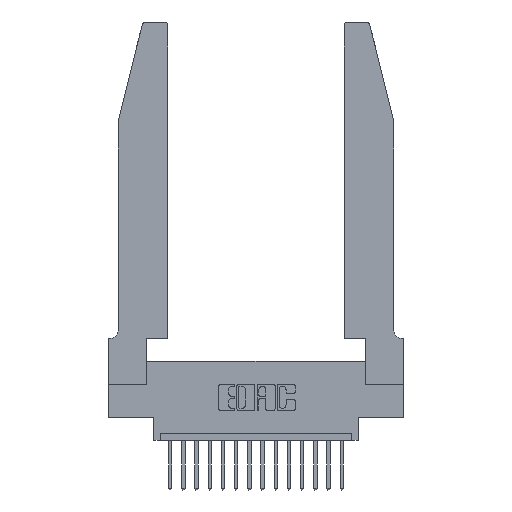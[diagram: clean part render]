
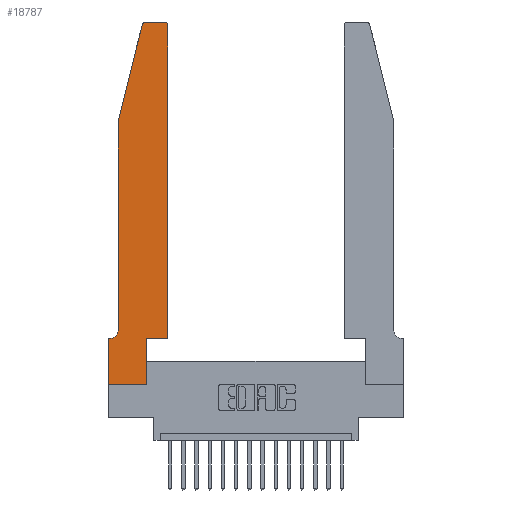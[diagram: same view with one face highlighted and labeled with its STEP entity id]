
A CAD part, top view. The second image highlights one B-rep face of the part: STEP entity #18787.
In plain terms, the highlighted planar face has unit normal (0, 0, 1).
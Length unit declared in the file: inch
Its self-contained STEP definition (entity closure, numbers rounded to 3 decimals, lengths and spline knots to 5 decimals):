
#164 = CARTESIAN_POINT ( 'NONE',  ( 0.2865, 0.35, 0.37 ) ) ;
#179 = LINE ( 'NONE', #12883, #6215 ) ;
#293 = ORIENTED_EDGE ( 'NONE', *, *, #19156, .T. ) ;
#517 = CARTESIAN_POINT ( 'NONE',  ( 0.0055, 0.35, 0.37 ) ) ;
#613 = LINE ( 'NONE', #4109, #13814 ) ;
#632 = LINE ( 'NONE', #2303, #2218 ) ;
#1124 = VERTEX_POINT ( 'NONE', #10151 ) ;
#1324 = LINE ( 'NONE', #10356, #12655 ) ;
#1396 = LINE ( 'NONE', #11299, #3714 ) ;
#1861 = VECTOR ( 'NONE', #18039, 39.37008 ) ;
#2035 = CARTESIAN_POINT ( 'NONE',  ( 0.0755, 2., 0.37 ) ) ;
#2218 = VECTOR ( 'NONE', #15643, 39.37008 ) ;
#2280 = DIRECTION ( 'NONE',  ( 1., 0., 0. ) ) ;
#2303 = CARTESIAN_POINT ( 'NONE',  ( 0., 0., 0.37 ) ) ;
#2309 = DIRECTION ( 'NONE',  ( 0., 1., 0. ) ) ;
#2317 = EDGE_CURVE ( 'NONE', #17494, #17172, #6606, .T. ) ;
#2878 = AXIS2_PLACEMENT_3D ( 'NONE', #15754, #18750, #2280 ) ;
#3079 = CARTESIAN_POINT ( 'NONE',  ( 0.0055, 0.42, 0.37 ) ) ;
#3263 = VERTEX_POINT ( 'NONE', #17427 ) ;
#3276 = AXIS2_PLACEMENT_3D ( 'NONE', #5026, #5150, #6595 ) ;
#3709 = ORIENTED_EDGE ( 'NONE', *, *, #2317, .T. ) ;
#3714 = VECTOR ( 'NONE', #14324, 39.37008 ) ;
#4109 = CARTESIAN_POINT ( 'NONE',  ( 0.0755, 2., 0.37 ) ) ;
#4634 = LINE ( 'NONE', #18600, #15256 ) ;
#4709 = CARTESIAN_POINT ( 'NONE',  ( 0.0755, 2., 0.37 ) ) ;
#4765 = EDGE_CURVE ( 'NONE', #7275, #1124, #8635, .T. ) ;
#4946 = CARTESIAN_POINT ( 'NONE',  ( 0.0755, 0.35, 0.37 ) ) ;
#5026 = CARTESIAN_POINT ( 'NONE',  ( 0.4205, 2.72, 0.37 ) ) ;
#5150 = DIRECTION ( 'NONE',  ( 0., 0., 1. ) ) ;
#5419 = CARTESIAN_POINT ( 'NONE',  ( 0., 0.35, 0.37 ) ) ;
#6215 = VECTOR ( 'NONE', #2309, 39.37008 ) ;
#6522 = ORIENTED_EDGE ( 'NONE', *, *, #7388, .T. ) ;
#6595 = DIRECTION ( 'NONE',  ( 1., 0., 0. ) ) ;
#6606 = LINE ( 'NONE', #4709, #18415 ) ;
#6623 = ORIENTED_EDGE ( 'NONE', *, *, #4765, .T. ) ;
#6627 = DIRECTION ( 'NONE',  ( 0., -1., 0. ) ) ;
#6651 = CIRCLE ( 'NONE', #7516, 0.07 ) ;
#6814 = DIRECTION ( 'NONE',  ( -1., 0., 0. ) ) ;
#6821 = EDGE_CURVE ( 'NONE', #17057, #7670, #17085, .T. ) ;
#7275 = VERTEX_POINT ( 'NONE', #9514 ) ;
#7388 = EDGE_CURVE ( 'NONE', #10219, #11679, #632, .T. ) ;
#7480 = ORIENTED_EDGE ( 'NONE', *, *, #8324, .T. ) ;
#7516 = AXIS2_PLACEMENT_3D ( 'NONE', #3079, #10395, #16140 ) ;
#7670 = VERTEX_POINT ( 'NONE', #7999 ) ;
#7853 = EDGE_CURVE ( 'NONE', #3263, #17057, #179, .T. ) ;
#7999 = CARTESIAN_POINT ( 'NONE',  ( 0.4205, 2.75, 0.37 ) ) ;
#8324 = EDGE_CURVE ( 'NONE', #17172, #9567, #6651, .T. ) ;
#8348 = LINE ( 'NONE', #164, #1861 ) ;
#8607 = CARTESIAN_POINT ( 'NONE',  ( 0.0755, 0.42, 0.37 ) ) ;
#8635 = CIRCLE ( 'NONE', #2878, 0.03 ) ;
#8718 = VECTOR ( 'NONE', #6814, 39.37008 ) ;
#8834 = DIRECTION ( 'NONE',  ( -0.239, -0.971, 0. ) ) ;
#9291 = AXIS2_PLACEMENT_3D ( 'NONE', #5419, #9832, #18762 ) ;
#9304 = ORIENTED_EDGE ( 'NONE', *, *, #17324, .T. ) ;
#9514 = CARTESIAN_POINT ( 'NONE',  ( 0.284, 2.75, 0.37 ) ) ;
#9567 = VERTEX_POINT ( 'NONE', #517 ) ;
#9832 = DIRECTION ( 'NONE',  ( 0., 0., 1. ) ) ;
#10151 = CARTESIAN_POINT ( 'NONE',  ( 0.25487, 2.72718, 0.37 ) ) ;
#10219 = VERTEX_POINT ( 'NONE', #12511 ) ;
#10356 = CARTESIAN_POINT ( 'NONE',  ( 0.2605, 2.75, 0.37 ) ) ;
#10395 = DIRECTION ( 'NONE',  ( 0., 0., -1. ) ) ;
#10877 = VERTEX_POINT ( 'NONE', #11639 ) ;
#11011 = EDGE_CURVE ( 'NONE', #18252, #3263, #1396, .T. ) ;
#11254 = PLANE ( 'NONE',  #9291 ) ;
#11299 = CARTESIAN_POINT ( 'NONE',  ( 0.4505, 0.35, 0.37 ) ) ;
#11639 = CARTESIAN_POINT ( 'NONE',  ( 0., 0.35, 0.37 ) ) ;
#11679 = VERTEX_POINT ( 'NONE', #12383 ) ;
#11720 = ORIENTED_EDGE ( 'NONE', *, *, #13647, .T. ) ;
#11757 = EDGE_CURVE ( 'NONE', #10877, #10219, #4634, .T. ) ;
#11895 = DIRECTION ( 'NONE',  ( -1., 0., 0. ) ) ;
#12014 = FACE_OUTER_BOUND ( 'NONE', #18721, .T. ) ;
#12111 = ORIENTED_EDGE ( 'NONE', *, *, #6821, .T. ) ;
#12190 = ORIENTED_EDGE ( 'NONE', *, *, #11011, .T. ) ;
#12383 = CARTESIAN_POINT ( 'NONE',  ( 0.2865, 0., 0.37 ) ) ;
#12511 = CARTESIAN_POINT ( 'NONE',  ( 0., 0., 0.37 ) ) ;
#12655 = VECTOR ( 'NONE', #11895, 39.37008 ) ;
#12883 = CARTESIAN_POINT ( 'NONE',  ( 0.4505, 0.35, 0.37 ) ) ;
#12939 = CARTESIAN_POINT ( 'NONE',  ( 0.4505, 2.72, 0.37 ) ) ;
#13647 = EDGE_CURVE ( 'NONE', #1124, #17494, #613, .T. ) ;
#13681 = DIRECTION ( 'NONE',  ( 0., -1., 0. ) ) ;
#13814 = VECTOR ( 'NONE', #8834, 39.37008 ) ;
#14007 = LINE ( 'NONE', #4946, #8718 ) ;
#14324 = DIRECTION ( 'NONE',  ( 1., 0., 0. ) ) ;
#14710 = EDGE_CURVE ( 'NONE', #9567, #10877, #14007, .T. ) ;
#14941 = ORIENTED_EDGE ( 'NONE', *, *, #11757, .T. ) ;
#15256 = VECTOR ( 'NONE', #6627, 39.37008 ) ;
#15643 = DIRECTION ( 'NONE',  ( 1., 0., 0. ) ) ;
#15653 = CARTESIAN_POINT ( 'NONE',  ( 0.2865, 0.35, 0.37 ) ) ;
#15754 = CARTESIAN_POINT ( 'NONE',  ( 0.284, 2.72, 0.37 ) ) ;
#16140 = DIRECTION ( 'NONE',  ( -1., 0., 0. ) ) ;
#16993 = ORIENTED_EDGE ( 'NONE', *, *, #7853, .T. ) ;
#17057 = VERTEX_POINT ( 'NONE', #12939 ) ;
#17085 = CIRCLE ( 'NONE', #3276, 0.03 ) ;
#17172 = VERTEX_POINT ( 'NONE', #8607 ) ;
#17324 = EDGE_CURVE ( 'NONE', #11679, #18252, #8348, .T. ) ;
#17427 = CARTESIAN_POINT ( 'NONE',  ( 0.4505, 0.35, 0.37 ) ) ;
#17494 = VERTEX_POINT ( 'NONE', #2035 ) ;
#17631 = ORIENTED_EDGE ( 'NONE', *, *, #14710, .T. ) ;
#18039 = DIRECTION ( 'NONE',  ( 0., 1., 0. ) ) ;
#18252 = VERTEX_POINT ( 'NONE', #15653 ) ;
#18415 = VECTOR ( 'NONE', #13681, 39.37008 ) ;
#18600 = CARTESIAN_POINT ( 'NONE',  ( 0., 0., 0.37 ) ) ;
#18721 = EDGE_LOOP ( 'NONE', ( #293, #6623, #11720, #3709, #7480, #17631, #14941, #6522, #9304, #12190, #16993, #12111 ) ) ;
#18750 = DIRECTION ( 'NONE',  ( 0., 0., 1. ) ) ;
#18762 = DIRECTION ( 'NONE',  ( 1., 0., 0. ) ) ;
#18787 = ADVANCED_FACE ( 'NONE', ( #12014 ), #11254, .T. ) ;
#19156 = EDGE_CURVE ( 'NONE', #7670, #7275, #1324, .T. ) ;
